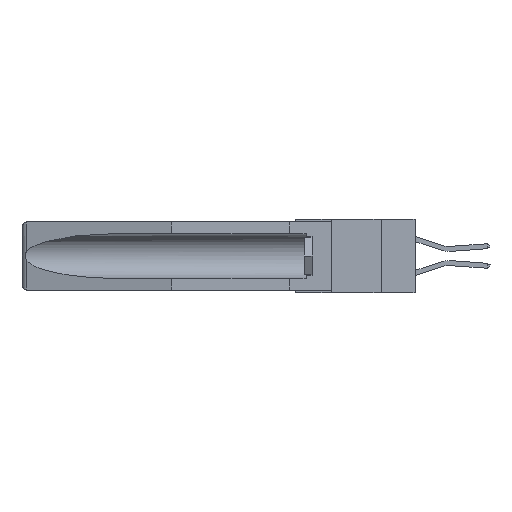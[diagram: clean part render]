
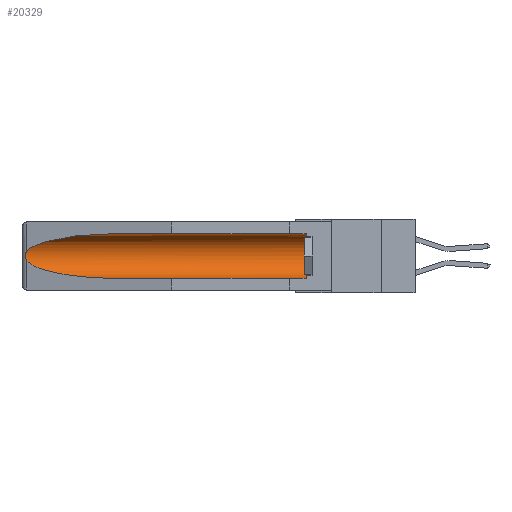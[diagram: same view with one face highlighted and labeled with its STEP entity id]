
A CAD part, left-side view. The second image highlights one B-rep face of the part: STEP entity #20329.
In plain terms, the highlighted cylindrical face has radius 2.857 mm (diameter 5.715 mm), a partial arc.
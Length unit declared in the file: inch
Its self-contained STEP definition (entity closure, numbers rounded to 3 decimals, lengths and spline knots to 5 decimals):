
#1 = EDGE_CURVE ( 'NONE', #6418, #18518, #19010, .T. ) ;
#70 = ORIENTED_EDGE ( 'NONE', *, *, #14666, .T. ) ;
#898 = CARTESIAN_POINT ( 'NONE',  ( 0.2673, 1.53269, -0.17917 ) ) ;
#985 = CARTESIAN_POINT ( 'NONE',  ( 0.2673, 1.5327, -0.16383 ) ) ;
#1019 = DIRECTION ( 'NONE',  ( 0., 1., 0. ) ) ;
#1668 = EDGE_CURVE ( 'NONE', #10316, #18683, #9121, .T. ) ;
#1951 = AXIS2_PLACEMENT_3D ( 'NONE', #17610, #2293, #9127 ) ;
#2082 = CARTESIAN_POINT ( 'NONE',  ( 0.25451, 1.48313, -0.09465 ) ) ;
#2265 = DIRECTION ( 'NONE',  ( 0., -1., 0. ) ) ;
#2293 = DIRECTION ( 'NONE',  ( 0., 1., 0. ) ) ;
#4019 = CARTESIAN_POINT ( 'NONE',  ( 0.26597, 1.52961, -0.15275 ) ) ;
#5213 =( BOUNDED_CURVE ( )  B_SPLINE_CURVE ( 3, ( #5971, #17670, #8085, #19782 ),
 .UNSPECIFIED., .F., .F. ) 
 B_SPLINE_CURVE_WITH_KNOTS ( ( 4, 4 ),
 ( 0.1948, 1.5708 ),
 .UNSPECIFIED. ) 
 CURVE ( )  GEOMETRIC_REPRESENTATION_ITEM ( )  RATIONAL_B_SPLINE_CURVE ( ( 1., 0.848, 0.848, 1. ) ) 
 REPRESENTATION_ITEM ( '' )  );
#5339 = VERTEX_POINT ( 'NONE', #17440 ) ;
#5970 = FACE_OUTER_BOUND ( 'NONE', #15808, .T. ) ;
#5971 = CARTESIAN_POINT ( 'NONE',  ( 0.26537, 1.52718, -0.19328 ) ) ;
#6066 = CARTESIAN_POINT ( 'NONE',  ( 0.26597, 1.5296, -0.19026 ) ) ;
#6418 = VERTEX_POINT ( 'NONE', #19521 ) ;
#6421 = CARTESIAN_POINT ( 'NONE',  ( 0.155, 1.07973, -0.059 ) ) ;
#6878 = ORIENTED_EDGE ( 'NONE', *, *, #9572, .T. ) ;
#7148 = CARTESIAN_POINT ( 'NONE',  ( 0.26537, 1.52718, -0.14972 ) ) ;
#7226 = CARTESIAN_POINT ( 'NONE',  ( 0.21114, 1.30732, -0.059 ) ) ;
#8085 = CARTESIAN_POINT ( 'NONE',  ( 0.21114, 1.30732, -0.284 ) ) ;
#8789 = VERTEX_POINT ( 'NONE', #13696 ) ;
#8821 = VECTOR ( 'NONE', #14186, 39.37008 ) ;
#8834 = CARTESIAN_POINT ( 'NONE',  ( 0.155, 1.07973, -0.059 ) ) ;
#9121 =( BOUNDED_CURVE ( )  B_SPLINE_CURVE ( 3, ( #8834, #7226, #2082, #7148 ),
 .UNSPECIFIED., .F., .F. ) 
 B_SPLINE_CURVE_WITH_KNOTS ( ( 4, 4 ),
 ( 4.71239, 6.08839 ),
 .UNSPECIFIED. ) 
 CURVE ( )  GEOMETRIC_REPRESENTATION_ITEM ( )  RATIONAL_B_SPLINE_CURVE ( ( 1., 0.848, 0.848, 1. ) ) 
 REPRESENTATION_ITEM ( '' )  );
#9127 = DIRECTION ( 'NONE',  ( 0., 0., 1. ) ) ;
#9286 = ORIENTED_EDGE ( 'NONE', *, *, #20491, .F. ) ;
#9572 = EDGE_CURVE ( 'NONE', #18683, #8789, #21449, .T. ) ;
#9654 = ORIENTED_EDGE ( 'NONE', *, *, #20259, .T. ) ;
#10316 = VERTEX_POINT ( 'NONE', #6421 ) ;
#10402 = VECTOR ( 'NONE', #1019, 39.37008 ) ;
#10950 = LINE ( 'NONE', #14485, #10402 ) ;
#10975 = CARTESIAN_POINT ( 'NONE',  ( 0.2675, 1.53308, -0.16763 ) ) ;
#11052 = CARTESIAN_POINT ( 'NONE',  ( 0.2675, 1.53308, -0.17534 ) ) ;
#12220 = DIRECTION ( 'NONE',  ( 0., 0., 1. ) ) ;
#12634 = CARTESIAN_POINT ( 'NONE',  ( 0.26537, 1.52718, -0.19328 ) ) ;
#13696 = CARTESIAN_POINT ( 'NONE',  ( 0.26537, 1.52718, -0.19328 ) ) ;
#14166 = ORIENTED_EDGE ( 'NONE', *, *, #1, .T. ) ;
#14186 = DIRECTION ( 'NONE',  ( 0., 1., 0. ) ) ;
#14355 = CARTESIAN_POINT ( 'NONE',  ( 0.26537, 1.52718, -0.14972 ) ) ;
#14485 = CARTESIAN_POINT ( 'NONE',  ( 0.155, -0.30754, -0.284 ) ) ;
#14666 = EDGE_CURVE ( 'NONE', #8789, #5339, #5213, .T. ) ;
#15592 = AXIS2_PLACEMENT_3D ( 'NONE', #20142, #2265, #12220 ) ;
#15808 = EDGE_LOOP ( 'NONE', ( #18986, #6878, #70, #9286, #14166, #9654 ) ) ;
#16459 = CYLINDRICAL_SURFACE ( 'NONE', #1951, 0.1125 ) ;
#16824 = CARTESIAN_POINT ( 'NONE',  ( 0.155, 0.126, -0.059 ) ) ;
#17440 = CARTESIAN_POINT ( 'NONE',  ( 0.155, 1.07973, -0.284 ) ) ;
#17610 = CARTESIAN_POINT ( 'NONE',  ( 0.155, -0.30754, -0.1715 ) ) ;
#17670 = CARTESIAN_POINT ( 'NONE',  ( 0.25451, 1.48313, -0.24835 ) ) ;
#18518 = VERTEX_POINT ( 'NONE', #16824 ) ;
#18683 = VERTEX_POINT ( 'NONE', #14355 ) ;
#18986 = ORIENTED_EDGE ( 'NONE', *, *, #1668, .T. ) ;
#18994 = CARTESIAN_POINT ( 'NONE',  ( 0.26537, 1.52718, -0.14972 ) ) ;
#19010 = CIRCLE ( 'NONE', #15592, 0.1125 ) ;
#19151 = CARTESIAN_POINT ( 'NONE',  ( 0.26654, 1.53092, -0.15636 ) ) ;
#19456 = CARTESIAN_POINT ( 'NONE',  ( 0.26655, 1.53094, -0.18657 ) ) ;
#19521 = CARTESIAN_POINT ( 'NONE',  ( 0.155, 0.126, -0.284 ) ) ;
#19782 = CARTESIAN_POINT ( 'NONE',  ( 0.155, 1.07973, -0.284 ) ) ;
#20142 = CARTESIAN_POINT ( 'NONE',  ( 0.155, 0.126, -0.1715 ) ) ;
#20259 = EDGE_CURVE ( 'NONE', #18518, #10316, #20351, .T. ) ;
#20329 = ADVANCED_FACE ( 'NONE', ( #5970 ), #16459, .F. ) ;
#20351 = LINE ( 'NONE', #20814, #8821 ) ;
#20491 = EDGE_CURVE ( 'NONE', #6418, #5339, #10950, .T. ) ;
#20814 = CARTESIAN_POINT ( 'NONE',  ( 0.155, -0.30754, -0.059 ) ) ;
#21449 = B_SPLINE_CURVE_WITH_KNOTS ( 'NONE', 3,
 ( #18994, #4019, #19151, #985, #10975, #11052, #898, #19456, #6066, #12634 ),
 .UNSPECIFIED., .F., .F.,
 ( 4, 2, 2, 2, 4 ),
 ( 0., 0.00029, 0.00058, 0.00087, 0.00117 ),
 .UNSPECIFIED. ) ;
